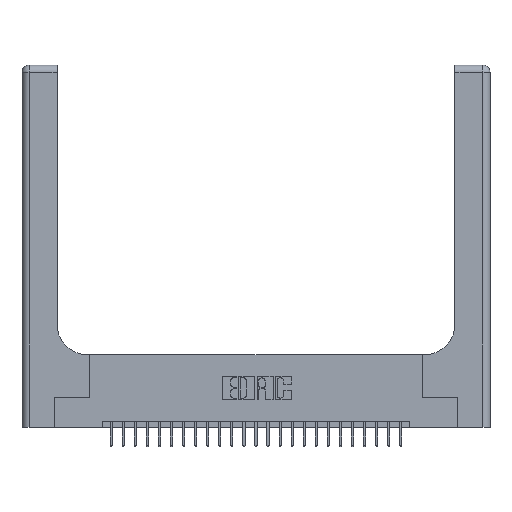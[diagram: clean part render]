
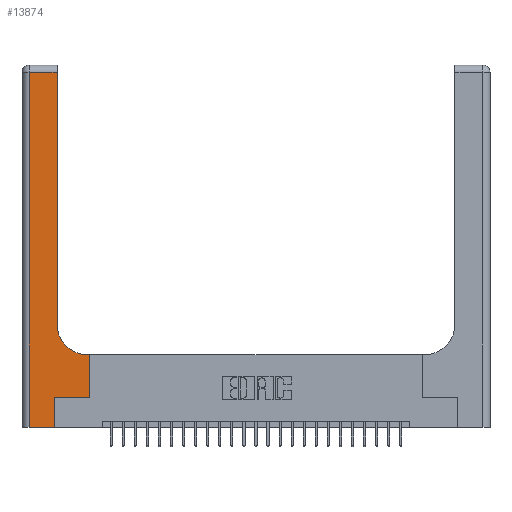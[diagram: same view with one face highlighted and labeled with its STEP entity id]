
A CAD part, top view. The second image highlights one B-rep face of the part: STEP entity #13874.
In plain terms, the highlighted planar face has unit normal (0, 0, 1).
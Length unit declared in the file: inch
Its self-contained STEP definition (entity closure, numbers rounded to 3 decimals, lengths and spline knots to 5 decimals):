
#1010 = VERTEX_POINT ( 'NONE', #6769 ) ;
#1183 = DIRECTION ( 'NONE',  ( -1., 0., 0. ) ) ;
#2010 = DIRECTION ( 'NONE',  ( 1., 0., 0. ) ) ;
#2113 = CARTESIAN_POINT ( 'NONE',  ( 0., 0., 0.37 ) ) ;
#2584 = ORIENTED_EDGE ( 'NONE', *, *, #25545, .T. ) ;
#3457 = EDGE_CURVE ( 'NONE', #13484, #9128, #22785, .T. ) ;
#3952 = LINE ( 'NONE', #7606, #25487 ) ;
#4431 = CARTESIAN_POINT ( 'NONE',  ( 0.5585, 0.25, 0.37 ) ) ;
#4733 = LINE ( 'NONE', #14627, #21350 ) ;
#4821 = CARTESIAN_POINT ( 'NONE',  ( 0.06, 2.94, 0.37 ) ) ;
#5369 = VECTOR ( 'NONE', #9900, 39.37008 ) ;
#5598 = LINE ( 'NONE', #14348, #16703 ) ;
#5635 = CARTESIAN_POINT ( 'NONE',  ( 0., 2.94, 0.37 ) ) ;
#5862 = VERTEX_POINT ( 'NONE', #23046 ) ;
#5924 = DIRECTION ( 'NONE',  ( 0., 1., 0. ) ) ;
#6171 = EDGE_LOOP ( 'NONE', ( #2584, #10119, #14080, #20895, #6438, #23814, #6930, #23543, #23316 ) ) ;
#6438 = ORIENTED_EDGE ( 'NONE', *, *, #25712, .T. ) ;
#6769 = CARTESIAN_POINT ( 'NONE',  ( 0.269, 0.25, 0.37 ) ) ;
#6930 = ORIENTED_EDGE ( 'NONE', *, *, #23500, .T. ) ;
#7606 = CARTESIAN_POINT ( 'NONE',  ( 0.2915, 3., 0.37 ) ) ;
#8365 = CARTESIAN_POINT ( 'NONE',  ( 0.269, 0., 0.37 ) ) ;
#8427 = VERTEX_POINT ( 'NONE', #20305 ) ;
#8616 = DIRECTION ( 'NONE',  ( 1., 0., 0. ) ) ;
#9128 = VERTEX_POINT ( 'NONE', #12484 ) ;
#9548 = LINE ( 'NONE', #4431, #10197 ) ;
#9756 = DIRECTION ( 'NONE',  ( 0., 1., 0. ) ) ;
#9900 = DIRECTION ( 'NONE',  ( -1., 0., 0. ) ) ;
#10014 = VERTEX_POINT ( 'NONE', #19501 ) ;
#10119 = ORIENTED_EDGE ( 'NONE', *, *, #21118, .T. ) ;
#10121 = LINE ( 'NONE', #2113, #26018 ) ;
#10197 = VECTOR ( 'NONE', #10780, 39.37008 ) ;
#10780 = DIRECTION ( 'NONE',  ( 0., 1., 0. ) ) ;
#11084 = EDGE_CURVE ( 'NONE', #8427, #25198, #10121, .T. ) ;
#11779 = CARTESIAN_POINT ( 'NONE',  ( 0.5415, 0.85, 0.37 ) ) ;
#12484 = CARTESIAN_POINT ( 'NONE',  ( 0.2915, 0.85, 0.37 ) ) ;
#13484 = VERTEX_POINT ( 'NONE', #24850 ) ;
#13844 = DIRECTION ( 'NONE',  ( 0., 0., -1. ) ) ;
#13856 = DIRECTION ( 'NONE',  ( 1., 0., 0. ) ) ;
#13874 = ADVANCED_FACE ( 'NONE', ( #26383 ), #26284, .F. ) ;
#14080 = ORIENTED_EDGE ( 'NONE', *, *, #20773, .T. ) ;
#14348 = CARTESIAN_POINT ( 'NONE',  ( 0.269, 0., 0.37 ) ) ;
#14524 = VECTOR ( 'NONE', #16404, 39.37008 ) ;
#14553 = LINE ( 'NONE', #25323, #19387 ) ;
#14627 = CARTESIAN_POINT ( 'NONE',  ( 0.269, 0.25, 0.37 ) ) ;
#16404 = DIRECTION ( 'NONE',  ( -1., 0., 0. ) ) ;
#16469 = LINE ( 'NONE', #5635, #5369 ) ;
#16703 = VECTOR ( 'NONE', #5924, 39.37008 ) ;
#19387 = VECTOR ( 'NONE', #23214, 39.37008 ) ;
#19501 = CARTESIAN_POINT ( 'NONE',  ( 0.2915, 2.94, 0.37 ) ) ;
#20027 = LINE ( 'NONE', #22549, #14524 ) ;
#20305 = CARTESIAN_POINT ( 'NONE',  ( 0.06, 0., 0.37 ) ) ;
#20690 = EDGE_CURVE ( 'NONE', #1010, #5862, #4733, .T. ) ;
#20773 = EDGE_CURVE ( 'NONE', #20844, #8427, #14553, .T. ) ;
#20844 = VERTEX_POINT ( 'NONE', #4821 ) ;
#20895 = ORIENTED_EDGE ( 'NONE', *, *, #11084, .T. ) ;
#21118 = EDGE_CURVE ( 'NONE', #10014, #20844, #16469, .T. ) ;
#21199 = EDGE_CURVE ( 'NONE', #21846, #13484, #20027, .T. ) ;
#21350 = VECTOR ( 'NONE', #2010, 39.37008 ) ;
#21846 = VERTEX_POINT ( 'NONE', #23365 ) ;
#22080 = CARTESIAN_POINT ( 'NONE',  ( 0., 3., 0.37 ) ) ;
#22549 = CARTESIAN_POINT ( 'NONE',  ( 0.2915, 0.6, 0.37 ) ) ;
#22785 = CIRCLE ( 'NONE', #23941, 0.25 ) ;
#23046 = CARTESIAN_POINT ( 'NONE',  ( 0.5585, 0.25, 0.37 ) ) ;
#23214 = DIRECTION ( 'NONE',  ( 0., -1., 0. ) ) ;
#23316 = ORIENTED_EDGE ( 'NONE', *, *, #3457, .T. ) ;
#23365 = CARTESIAN_POINT ( 'NONE',  ( 0.5585, 0.6, 0.37 ) ) ;
#23500 = EDGE_CURVE ( 'NONE', #5862, #21846, #9548, .T. ) ;
#23543 = ORIENTED_EDGE ( 'NONE', *, *, #21199, .T. ) ;
#23814 = ORIENTED_EDGE ( 'NONE', *, *, #20690, .T. ) ;
#23941 = AXIS2_PLACEMENT_3D ( 'NONE', #11779, #26295, #13856 ) ;
#24850 = CARTESIAN_POINT ( 'NONE',  ( 0.5415, 0.6, 0.37 ) ) ;
#25198 = VERTEX_POINT ( 'NONE', #8365 ) ;
#25323 = CARTESIAN_POINT ( 'NONE',  ( 0.06, 3., 0.37 ) ) ;
#25487 = VECTOR ( 'NONE', #9756, 39.37008 ) ;
#25545 = EDGE_CURVE ( 'NONE', #9128, #10014, #3952, .T. ) ;
#25712 = EDGE_CURVE ( 'NONE', #25198, #1010, #5598, .T. ) ;
#26018 = VECTOR ( 'NONE', #8616, 39.37008 ) ;
#26284 = PLANE ( 'NONE',  #27106 ) ;
#26295 = DIRECTION ( 'NONE',  ( 0., 0., -1. ) ) ;
#26383 = FACE_OUTER_BOUND ( 'NONE', #6171, .T. ) ;
#27106 = AXIS2_PLACEMENT_3D ( 'NONE', #22080, #13844, #1183 ) ;
